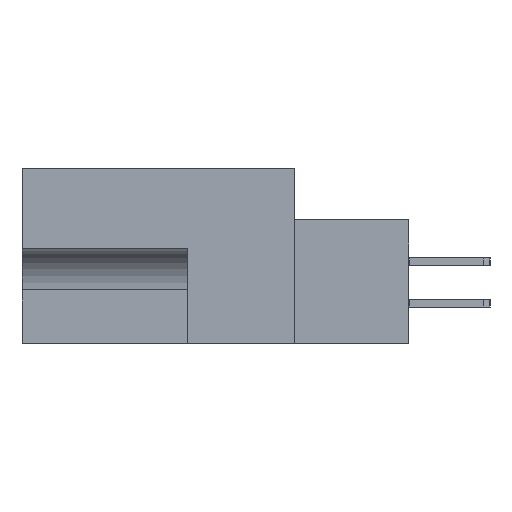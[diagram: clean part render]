
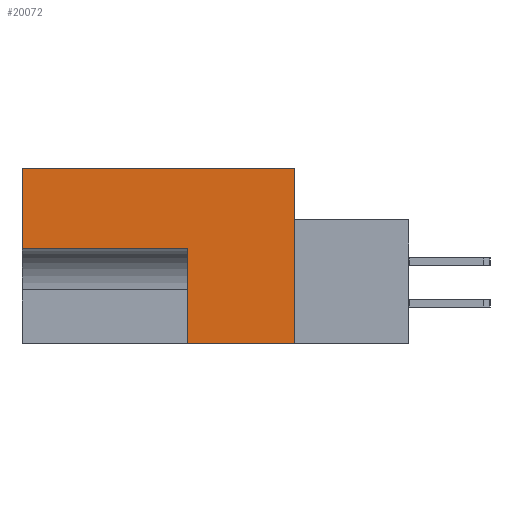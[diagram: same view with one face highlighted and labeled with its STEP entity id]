
A CAD part, left-side view. The second image highlights one B-rep face of the part: STEP entity #20072.
In plain terms, the highlighted planar face has unit normal (-1, 0, 0).
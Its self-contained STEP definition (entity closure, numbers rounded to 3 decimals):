
#30033 = EDGE_CURVE ( 'NONE', #20754, #2038, #4492, .T. ) ;
#1720 = CARTESIAN_POINT ( 'NONE',  ( 0., 20.955, 0. ) ) ;
#2038 = VERTEX_POINT ( 'NONE', #13627 ) ;
#2392 = DIRECTION ( 'NONE',  ( 0., 1., 0. ) ) ;
#2527 = EDGE_CURVE ( 'NONE', #6115, #21026, #23186, .T. ) ;
#2543 = FACE_OUTER_BOUND ( 'NONE', #23739, .T. ) ;
#4492 = LINE ( 'NONE', #23652, #16421 ) ;
#5699 = ORIENTED_EDGE ( 'NONE', *, *, #9040, .F. ) ;
#6115 = VERTEX_POINT ( 'NONE', #25912 ) ;
#6661 = CARTESIAN_POINT ( 'NONE',  ( 0., 0., 0. ) ) ;
#6699 = LINE ( 'NONE', #23358, #13891 ) ;
#7801 = CARTESIAN_POINT ( 'NONE',  ( 0., 8.255, -6.172 ) ) ;
#8142 = VERTEX_POINT ( 'NONE', #13783 ) ;
#9040 = EDGE_CURVE ( 'NONE', #2038, #6115, #25282, .T. ) ;
#10068 = DIRECTION ( 'NONE',  ( 0., 0., 1. ) ) ;
#10526 = CARTESIAN_POINT ( 'NONE',  ( 0., 0., 0. ) ) ;
#12836 = ORIENTED_EDGE ( 'NONE', *, *, #30033, .F. ) ;
#13182 = ORIENTED_EDGE ( 'NONE', *, *, #14584, .F. ) ;
#13605 = DIRECTION ( 'NONE',  ( 0., 0., 1. ) ) ;
#13627 = CARTESIAN_POINT ( 'NONE',  ( 0., 8.255, -6.172 ) ) ;
#13783 = CARTESIAN_POINT ( 'NONE',  ( 0., 0., -13.487 ) ) ;
#13891 = VECTOR ( 'NONE', #14088, 1000. ) ;
#14088 = DIRECTION ( 'NONE',  ( 0., 0., -1. ) ) ;
#14389 = VECTOR ( 'NONE', #2392, 1000. ) ;
#14584 = EDGE_CURVE ( 'NONE', #8142, #20754, #26015, .T. ) ;
#15304 = LINE ( 'NONE', #15605, #20775 ) ;
#15605 = CARTESIAN_POINT ( 'NONE',  ( 0., 11.506, 0. ) ) ;
#16218 = CARTESIAN_POINT ( 'NONE',  ( 0., -8.814, -13.487 ) ) ;
#16421 = VECTOR ( 'NONE', #10068, 1000. ) ;
#17103 = DIRECTION ( 'NONE',  ( 0., 1., 0. ) ) ;
#17472 = EDGE_CURVE ( 'NONE', #28073, #8142, #6699, .T. ) ;
#20072 = ADVANCED_FACE ( 'NONE', ( #2543 ), #20316, .F. ) ;
#20316 = PLANE ( 'NONE',  #24218 ) ;
#20562 = VECTOR ( 'NONE', #17103, 1000. ) ;
#20600 = ORIENTED_EDGE ( 'NONE', *, *, #25514, .F. ) ;
#20754 = VERTEX_POINT ( 'NONE', #26518 ) ;
#20775 = VECTOR ( 'NONE', #28136, 1000. ) ;
#21026 = VERTEX_POINT ( 'NONE', #1720 ) ;
#22563 = DIRECTION ( 'NONE',  ( 1., 0., 0. ) ) ;
#23186 = LINE ( 'NONE', #25201, #29332 ) ;
#23358 = CARTESIAN_POINT ( 'NONE',  ( 0., 0., 0. ) ) ;
#23652 = CARTESIAN_POINT ( 'NONE',  ( 0., 8.255, -13.487 ) ) ;
#23739 = EDGE_LOOP ( 'NONE', ( #13182, #25797, #20600, #28080, #5699, #12836 ) ) ;
#24218 = AXIS2_PLACEMENT_3D ( 'NONE', #6661, #22563, #24980 ) ;
#24980 = DIRECTION ( 'NONE',  ( 0., 0., -1. ) ) ;
#25201 = CARTESIAN_POINT ( 'NONE',  ( 0., 20.955, -13.487 ) ) ;
#25282 = LINE ( 'NONE', #7801, #20562 ) ;
#25514 = EDGE_CURVE ( 'NONE', #21026, #28073, #15304, .T. ) ;
#25797 = ORIENTED_EDGE ( 'NONE', *, *, #17472, .F. ) ;
#25912 = CARTESIAN_POINT ( 'NONE',  ( 0., 20.955, -6.172 ) ) ;
#26015 = LINE ( 'NONE', #16218, #14389 ) ;
#26518 = CARTESIAN_POINT ( 'NONE',  ( 0., 8.255, -13.487 ) ) ;
#28073 = VERTEX_POINT ( 'NONE', #10526 ) ;
#28080 = ORIENTED_EDGE ( 'NONE', *, *, #2527, .F. ) ;
#28136 = DIRECTION ( 'NONE',  ( 0., -1., 0. ) ) ;
#29332 = VECTOR ( 'NONE', #13605, 1000. ) ;
